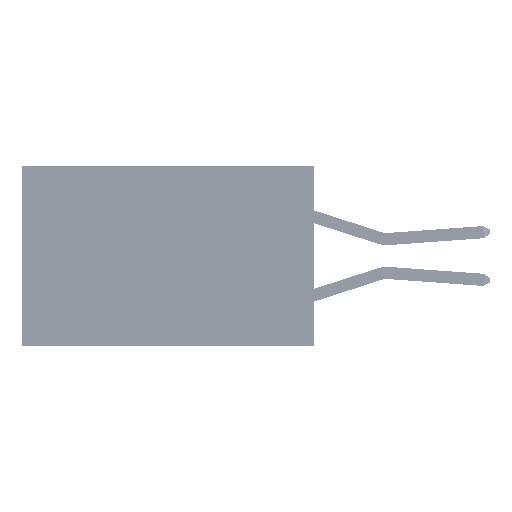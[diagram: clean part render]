
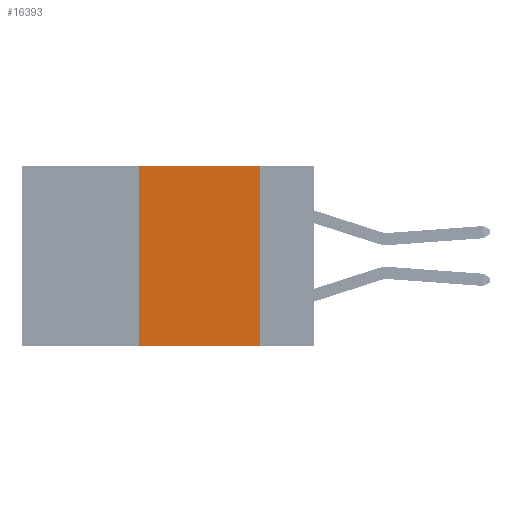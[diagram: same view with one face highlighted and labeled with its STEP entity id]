
A CAD part, left-side view. The second image highlights one B-rep face of the part: STEP entity #16393.
In plain terms, the highlighted planar face has unit normal (-1, 0, 0).
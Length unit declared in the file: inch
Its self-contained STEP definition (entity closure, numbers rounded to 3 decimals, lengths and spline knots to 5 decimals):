
#4841 = CARTESIAN_POINT ( 'NONE',  ( 0., 0.11, -0.37 ) ) ;
#5373 = CARTESIAN_POINT ( 'NONE',  ( 0., 0.6, 0. ) ) ;
#7453 = VERTEX_POINT ( 'NONE', #14180 ) ;
#8542 = VECTOR ( 'NONE', #34329, 39.37008 ) ;
#9619 = DIRECTION ( 'NONE',  ( 1., 0., 0. ) ) ;
#10149 = LINE ( 'NONE', #18126, #8542 ) ;
#10419 = CARTESIAN_POINT ( 'NONE',  ( 0., 0.36, 0. ) ) ;
#14180 = CARTESIAN_POINT ( 'NONE',  ( 0., 0.36, 0. ) ) ;
#15735 = ORIENTED_EDGE ( 'NONE', *, *, #46323, .F. ) ;
#16393 = ADVANCED_FACE ( 'NONE', ( #33292 ), #33549, .F. ) ;
#17946 = EDGE_CURVE ( 'NONE', #40152, #28271, #10149, .T. ) ;
#18126 = CARTESIAN_POINT ( 'NONE',  ( 0., 0.11, 0. ) ) ;
#18271 = LINE ( 'NONE', #42196, #32557 ) ;
#19440 = AXIS2_PLACEMENT_3D ( 'NONE', #5373, #9619, #20819 ) ;
#20819 = DIRECTION ( 'NONE',  ( 0., 0., -1. ) ) ;
#22238 = ORIENTED_EDGE ( 'NONE', *, *, #17946, .F. ) ;
#25593 = LINE ( 'NONE', #41512, #51702 ) ;
#27473 = VERTEX_POINT ( 'NONE', #50644 ) ;
#28271 = VERTEX_POINT ( 'NONE', #4841 ) ;
#31151 = LINE ( 'NONE', #10419, #44978 ) ;
#31373 = ORIENTED_EDGE ( 'NONE', *, *, #39370, .T. ) ;
#32557 = VECTOR ( 'NONE', #38196, 39.37008 ) ;
#33292 = FACE_OUTER_BOUND ( 'NONE', #46631, .T. ) ;
#33549 = PLANE ( 'NONE',  #19440 ) ;
#34329 = DIRECTION ( 'NONE',  ( 0., 0., -1. ) ) ;
#36213 = ORIENTED_EDGE ( 'NONE', *, *, #51183, .F. ) ;
#38196 = DIRECTION ( 'NONE',  ( 0., -1., 0. ) ) ;
#39370 = EDGE_CURVE ( 'NONE', #27473, #28271, #25593, .T. ) ;
#40152 = VERTEX_POINT ( 'NONE', #42469 ) ;
#41512 = CARTESIAN_POINT ( 'NONE',  ( 0., 0.6, -0.37 ) ) ;
#42196 = CARTESIAN_POINT ( 'NONE',  ( 0., 0.6, 0. ) ) ;
#42469 = CARTESIAN_POINT ( 'NONE',  ( 0., 0.11, 0. ) ) ;
#44978 = VECTOR ( 'NONE', #47352, 39.37008 ) ;
#46323 = EDGE_CURVE ( 'NONE', #7453, #40152, #18271, .T. ) ;
#46631 = EDGE_LOOP ( 'NONE', ( #22238, #15735, #36213, #31373 ) ) ;
#47352 = DIRECTION ( 'NONE',  ( 0., 0., 1. ) ) ;
#49215 = DIRECTION ( 'NONE',  ( 0., -1., 0. ) ) ;
#50644 = CARTESIAN_POINT ( 'NONE',  ( 0., 0.36, -0.37 ) ) ;
#51183 = EDGE_CURVE ( 'NONE', #27473, #7453, #31151, .T. ) ;
#51702 = VECTOR ( 'NONE', #49215, 39.37008 ) ;
